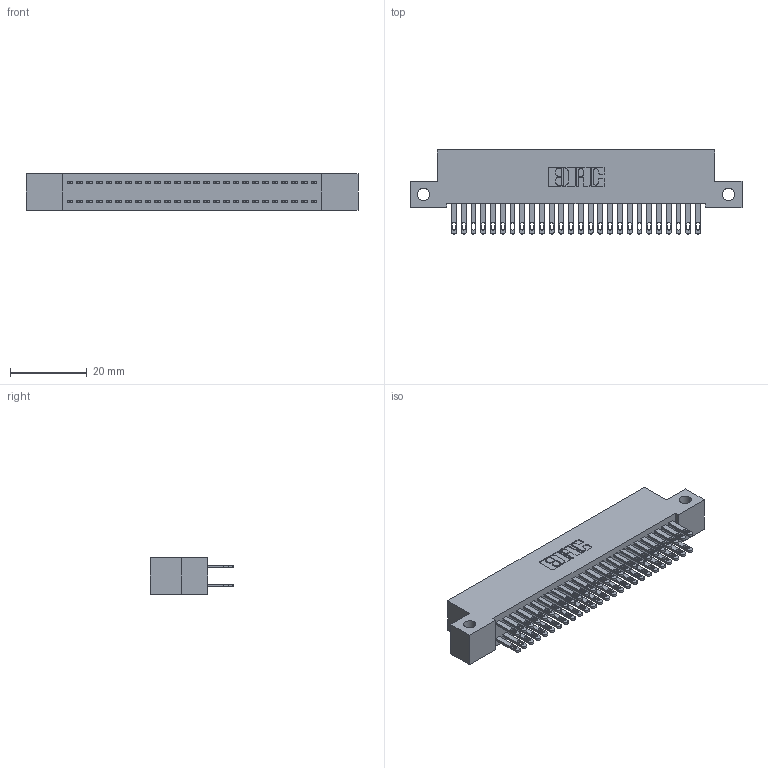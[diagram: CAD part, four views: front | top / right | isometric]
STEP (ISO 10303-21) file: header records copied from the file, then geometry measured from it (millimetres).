
FILE_DESCRIPTION (( 'STEP AP203' ), '1' );
FILE_NAME ('892-052-500-212.STEP', '2020-09-21T18:11:14', ( '' ), ( '' ), 'SwSTEP 2.0', 'SolidWorks 2020', '' );
FILE_SCHEMA (( 'CONFIG_CONTROL_DESIGN' ));
Length unit declared in the file: inch
Products named in the file (3): 345-292-001_345-293-100; 892-052-500-212; 842 Part_Side Mount
Assembly tree (53 placements, depth 2):
  892-052-500-212
    842 Part_Side Mount
    345-292-001_345-293-100  x52
Bounding box: 86.36 x 21.85 x 9.4 mm (x, y, z)
Volume: 7768.7 mm3; surface area: 12589.3 mm2
Topology: 53 solids, 53 shells, 2606 faces, 7943 edges, 5294 vertices
Faces by surface type: plane 1626, cylinder 980
Entity records: 18597 total; most frequent: CARTESIAN_POINT 3098, ORIENTED_EDGE 3034, DIRECTION 2677, EDGE_CURVE 1517, VECTOR 1385, LINE 1385, VERTEX_POINT 1010, AXIS2_PLACEMENT_3D 646
